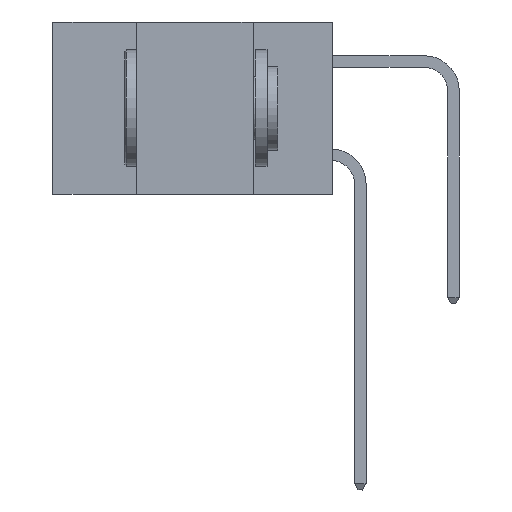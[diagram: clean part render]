
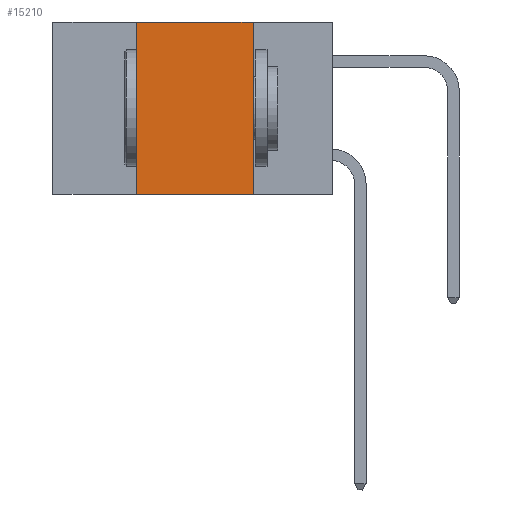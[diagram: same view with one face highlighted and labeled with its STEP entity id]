
A CAD part, left-side view. The second image highlights one B-rep face of the part: STEP entity #15210.
In plain terms, the highlighted planar face has unit normal (-1, 0, 0).
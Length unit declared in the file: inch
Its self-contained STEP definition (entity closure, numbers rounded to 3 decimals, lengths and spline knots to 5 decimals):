
#11 = VERTEX_POINT ( 'NONE', #12766 ) ;
#36 = EDGE_CURVE ( 'NONE', #16402, #11, #19563, .T. ) ;
#64 = EDGE_CURVE ( 'NONE', #3877, #8705, #2347, .T. ) ;
#1029 = VECTOR ( 'NONE', #18005, 39.37008 ) ;
#1501 = CARTESIAN_POINT ( 'NONE',  ( 0., 0.42, 0. ) ) ;
#2347 = LINE ( 'NONE', #12816, #6679 ) ;
#3877 = VERTEX_POINT ( 'NONE', #1501 ) ;
#4352 = CARTESIAN_POINT ( 'NONE',  ( 0., 0.42, -0.37 ) ) ;
#4880 = CARTESIAN_POINT ( 'NONE',  ( 0., 0.17, 0. ) ) ;
#6304 = PLANE ( 'NONE',  #11750 ) ;
#6679 = VECTOR ( 'NONE', #12920, 39.37008 ) ;
#7407 = ORIENTED_EDGE ( 'NONE', *, *, #17838, .F. ) ;
#7646 = ORIENTED_EDGE ( 'NONE', *, *, #64, .F. ) ;
#7873 = LINE ( 'NONE', #15852, #11668 ) ;
#7990 = DIRECTION ( 'NONE',  ( 1., 0., 0. ) ) ;
#8185 = ORIENTED_EDGE ( 'NONE', *, *, #11406, .F. ) ;
#8366 = ORIENTED_EDGE ( 'NONE', *, *, #36, .T. ) ;
#8705 = VERTEX_POINT ( 'NONE', #4880 ) ;
#9763 = LINE ( 'NONE', #18079, #1029 ) ;
#11406 = EDGE_CURVE ( 'NONE', #16402, #3877, #9763, .T. ) ;
#11668 = VECTOR ( 'NONE', #17449, 39.37008 ) ;
#11750 = AXIS2_PLACEMENT_3D ( 'NONE', #12800, #7990, #19237 ) ;
#12650 = CARTESIAN_POINT ( 'NONE',  ( 0., 0.6, -0.37 ) ) ;
#12766 = CARTESIAN_POINT ( 'NONE',  ( 0., 0.17, -0.37 ) ) ;
#12800 = CARTESIAN_POINT ( 'NONE',  ( 0., 0.6, 0. ) ) ;
#12816 = CARTESIAN_POINT ( 'NONE',  ( 0., 0.6, 0. ) ) ;
#12920 = DIRECTION ( 'NONE',  ( 0., -1., 0. ) ) ;
#13676 = DIRECTION ( 'NONE',  ( 0., -1., 0. ) ) ;
#15210 = ADVANCED_FACE ( 'NONE', ( #18277 ), #6304, .F. ) ;
#15852 = CARTESIAN_POINT ( 'NONE',  ( 0., 0.17, 0. ) ) ;
#16402 = VERTEX_POINT ( 'NONE', #4352 ) ;
#17181 = EDGE_LOOP ( 'NONE', ( #7407, #7646, #8185, #8366 ) ) ;
#17449 = DIRECTION ( 'NONE',  ( 0., 0., -1. ) ) ;
#17838 = EDGE_CURVE ( 'NONE', #8705, #11, #7873, .T. ) ;
#18005 = DIRECTION ( 'NONE',  ( 0., 0., 1. ) ) ;
#18079 = CARTESIAN_POINT ( 'NONE',  ( 0., 0.42, 0. ) ) ;
#18277 = FACE_OUTER_BOUND ( 'NONE', #17181, .T. ) ;
#19044 = VECTOR ( 'NONE', #13676, 39.37008 ) ;
#19237 = DIRECTION ( 'NONE',  ( 0., 0., -1. ) ) ;
#19563 = LINE ( 'NONE', #12650, #19044 ) ;
